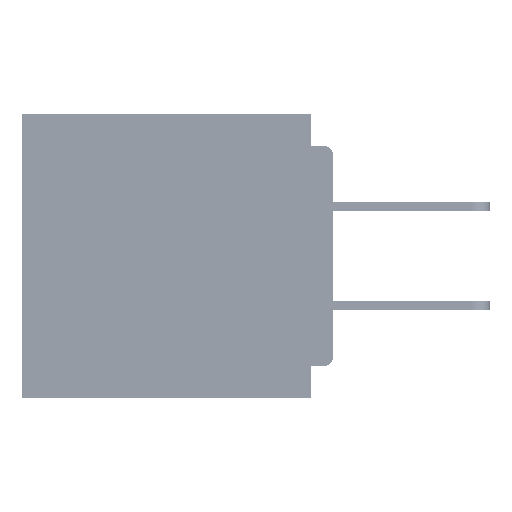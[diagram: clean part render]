
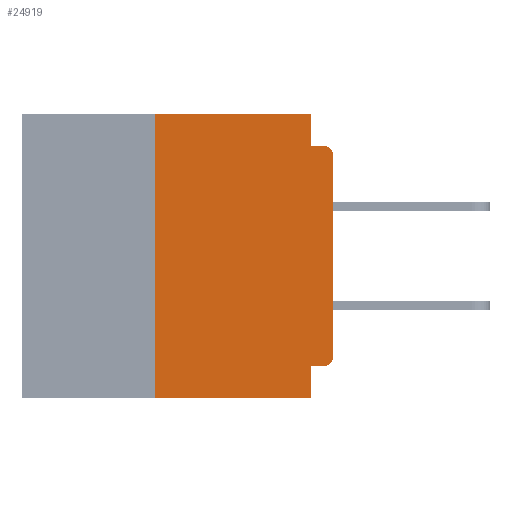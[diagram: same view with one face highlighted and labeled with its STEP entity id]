
A CAD part, left-side view. The second image highlights one B-rep face of the part: STEP entity #24919.
In plain terms, the highlighted planar face has unit normal (-1, 0, 0).
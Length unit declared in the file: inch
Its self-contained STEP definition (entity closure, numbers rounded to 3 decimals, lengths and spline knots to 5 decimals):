
#344 = EDGE_LOOP ( 'NONE', ( #45779, #23761, #15965, #55007, #27491, #49155, #19720, #4398, #5302, #27795 ) ) ;
#515 = CARTESIAN_POINT ( 'NONE',  ( 0., 0.031, 0. ) ) ;
#3021 = CIRCLE ( 'NONE', #41900, 0.015 ) ;
#3026 = VERTEX_POINT ( 'NONE', #31989 ) ;
#3630 = VERTEX_POINT ( 'NONE', #9583 ) ;
#4398 = ORIENTED_EDGE ( 'NONE', *, *, #9379, .F. ) ;
#5302 = ORIENTED_EDGE ( 'NONE', *, *, #28578, .F. ) ;
#5305 = DIRECTION ( 'NONE',  ( -1., 0., 0. ) ) ;
#5582 = AXIS2_PLACEMENT_3D ( 'NONE', #7928, #59770, #31638 ) ;
#6025 = VECTOR ( 'NONE', #56099, 39.37008 ) ;
#6195 = FACE_OUTER_BOUND ( 'NONE', #344, .T. ) ;
#7928 = CARTESIAN_POINT ( 'NONE',  ( 0., 0.437, 0. ) ) ;
#9379 = EDGE_CURVE ( 'NONE', #3026, #3630, #9473, .T. ) ;
#9473 = LINE ( 'NONE', #18441, #20526 ) ;
#9583 = CARTESIAN_POINT ( 'NONE',  ( 0., 0.031, -0.4 ) ) ;
#10932 = VECTOR ( 'NONE', #60611, 39.37008 ) ;
#11711 = EDGE_CURVE ( 'NONE', #20170, #48964, #46046, .T. ) ;
#11893 = CARTESIAN_POINT ( 'NONE',  ( 0., 0.25, -0.4 ) ) ;
#12445 = CARTESIAN_POINT ( 'NONE',  ( 0., 0., -0.06 ) ) ;
#12500 = VERTEX_POINT ( 'NONE', #33794 ) ;
#15301 = CARTESIAN_POINT ( 'NONE',  ( 0., 0., 0. ) ) ;
#15706 = VERTEX_POINT ( 'NONE', #22293 ) ;
#15965 = ORIENTED_EDGE ( 'NONE', *, *, #23010, .F. ) ;
#16547 = CARTESIAN_POINT ( 'NONE',  ( 0., 0., -0.355 ) ) ;
#18441 = CARTESIAN_POINT ( 'NONE',  ( 0., 0.031, -0.4 ) ) ;
#18960 = LINE ( 'NONE', #15301, #30059 ) ;
#19057 = CARTESIAN_POINT ( 'NONE',  ( 0., 0.25, -0.4 ) ) ;
#19720 = ORIENTED_EDGE ( 'NONE', *, *, #44297, .T. ) ;
#19842 = DIRECTION ( 'NONE',  ( 0., 0., 1. ) ) ;
#20170 = VERTEX_POINT ( 'NONE', #43717 ) ;
#20257 = CARTESIAN_POINT ( 'NONE',  ( 0., 0.015, -0.34 ) ) ;
#20338 = EDGE_CURVE ( 'NONE', #56310, #20170, #42183, .T. ) ;
#20526 = VECTOR ( 'NONE', #51359, 39.37008 ) ;
#21284 = DIRECTION ( 'NONE',  ( 0., 1., 0. ) ) ;
#21614 = LINE ( 'NONE', #40145, #45244 ) ;
#22293 = CARTESIAN_POINT ( 'NONE',  ( 0., 0.015, -0.355 ) ) ;
#22992 = CARTESIAN_POINT ( 'NONE',  ( 0., 0., -0.045 ) ) ;
#23010 = EDGE_CURVE ( 'NONE', #60200, #12500, #59538, .T. ) ;
#23761 = ORIENTED_EDGE ( 'NONE', *, *, #46425, .T. ) ;
#24919 = ADVANCED_FACE ( 'NONE', ( #6195 ), #26913, .F. ) ;
#25014 = DIRECTION ( 'NONE',  ( 0., 0., -1. ) ) ;
#26913 = PLANE ( 'NONE',  #5582 ) ;
#27491 = ORIENTED_EDGE ( 'NONE', *, *, #11711, .F. ) ;
#27795 = ORIENTED_EDGE ( 'NONE', *, *, #59699, .T. ) ;
#28168 = CARTESIAN_POINT ( 'NONE',  ( 0., 0., -0.34 ) ) ;
#28578 = EDGE_CURVE ( 'NONE', #15706, #3026, #33891, .T. ) ;
#29675 = VECTOR ( 'NONE', #54302, 39.37008 ) ;
#30059 = VECTOR ( 'NONE', #19842, 39.37008 ) ;
#30072 = VERTEX_POINT ( 'NONE', #12445 ) ;
#30742 = CIRCLE ( 'NONE', #32161, 0.015 ) ;
#31638 = DIRECTION ( 'NONE',  ( 0., 0., -1. ) ) ;
#31989 = CARTESIAN_POINT ( 'NONE',  ( 0., 0.031, -0.355 ) ) ;
#32161 = AXIS2_PLACEMENT_3D ( 'NONE', #20257, #53175, #25014 ) ;
#32421 = VECTOR ( 'NONE', #21284, 39.37008 ) ;
#32582 = LINE ( 'NONE', #51381, #6025 ) ;
#33493 = VECTOR ( 'NONE', #46217, 39.37008 ) ;
#33519 = CARTESIAN_POINT ( 'NONE',  ( 0., 0.015, -0.06 ) ) ;
#33794 = CARTESIAN_POINT ( 'NONE',  ( 0., 0.015, -0.045 ) ) ;
#33891 = LINE ( 'NONE', #16547, #32421 ) ;
#38268 = DIRECTION ( 'NONE',  ( 0., 0., -1. ) ) ;
#40145 = CARTESIAN_POINT ( 'NONE',  ( 0., 0.437, -0.4 ) ) ;
#41900 = AXIS2_PLACEMENT_3D ( 'NONE', #33519, #5305, #38268 ) ;
#42183 = LINE ( 'NONE', #11893, #29675 ) ;
#43139 = EDGE_CURVE ( 'NONE', #56250, #30072, #18960, .T. ) ;
#43717 = CARTESIAN_POINT ( 'NONE',  ( 0., 0.25, 0. ) ) ;
#44297 = EDGE_CURVE ( 'NONE', #56310, #3630, #21614, .T. ) ;
#45244 = VECTOR ( 'NONE', #49581, 39.37008 ) ;
#45779 = ORIENTED_EDGE ( 'NONE', *, *, #43139, .T. ) ;
#46046 = LINE ( 'NONE', #60135, #33493 ) ;
#46217 = DIRECTION ( 'NONE',  ( 0., -1., 0. ) ) ;
#46425 = EDGE_CURVE ( 'NONE', #30072, #12500, #3021, .T. ) ;
#48964 = VERTEX_POINT ( 'NONE', #515 ) ;
#49155 = ORIENTED_EDGE ( 'NONE', *, *, #20338, .F. ) ;
#49581 = DIRECTION ( 'NONE',  ( 0., -1., 0. ) ) ;
#51359 = DIRECTION ( 'NONE',  ( 0., 0., -1. ) ) ;
#51381 = CARTESIAN_POINT ( 'NONE',  ( 0., 0.031, 0. ) ) ;
#52523 = EDGE_CURVE ( 'NONE', #48964, #60200, #32582, .T. ) ;
#53175 = DIRECTION ( 'NONE',  ( -1., 0., 0. ) ) ;
#54302 = DIRECTION ( 'NONE',  ( 0., 0., 1. ) ) ;
#55007 = ORIENTED_EDGE ( 'NONE', *, *, #52523, .F. ) ;
#56099 = DIRECTION ( 'NONE',  ( 0., 0., -1. ) ) ;
#56250 = VERTEX_POINT ( 'NONE', #28168 ) ;
#56310 = VERTEX_POINT ( 'NONE', #19057 ) ;
#56591 = CARTESIAN_POINT ( 'NONE',  ( 0., 0.031, -0.045 ) ) ;
#59538 = LINE ( 'NONE', #22992, #10932 ) ;
#59699 = EDGE_CURVE ( 'NONE', #15706, #56250, #30742, .T. ) ;
#59770 = DIRECTION ( 'NONE',  ( 1., 0., 0. ) ) ;
#60135 = CARTESIAN_POINT ( 'NONE',  ( 0., 0.437, 0. ) ) ;
#60200 = VERTEX_POINT ( 'NONE', #56591 ) ;
#60611 = DIRECTION ( 'NONE',  ( 0., -1., 0. ) ) ;
